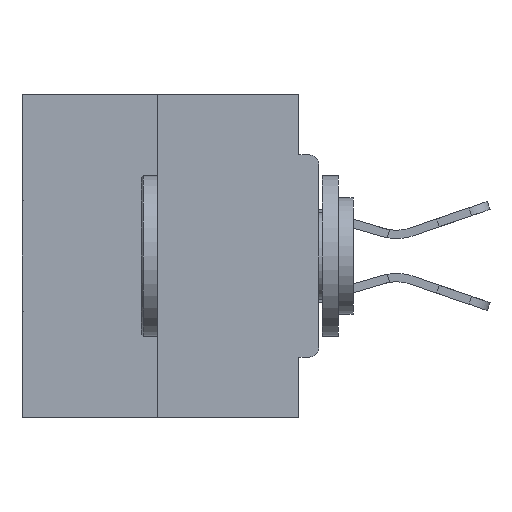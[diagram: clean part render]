
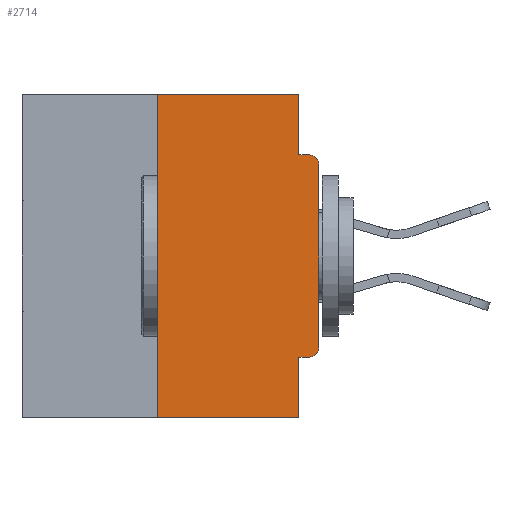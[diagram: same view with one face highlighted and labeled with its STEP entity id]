
A CAD part, left-side view. The second image highlights one B-rep face of the part: STEP entity #2714.
In plain terms, the highlighted planar face has unit normal (-1, 0, 0).
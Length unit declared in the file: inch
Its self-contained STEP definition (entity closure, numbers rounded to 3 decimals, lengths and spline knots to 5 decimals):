
#482 = CARTESIAN_POINT ( 'NONE',  ( 0., 0.25, 0. ) ) ;
#554 = LINE ( 'NONE', #13754, #11994 ) ;
#1395 = CARTESIAN_POINT ( 'NONE',  ( 0., 0.031, -0.4065 ) ) ;
#1674 = EDGE_CURVE ( 'NONE', #18976, #32118, #11681, .T. ) ;
#1680 = AXIS2_PLACEMENT_3D ( 'NONE', #21008, #1879, #27408 ) ;
#1879 = DIRECTION ( 'NONE',  ( -1., 0., 0. ) ) ;
#2221 = VECTOR ( 'NONE', #25900, 39.37008 ) ;
#2714 = ADVANCED_FACE ( 'NONE', ( #7146 ), #31697, .F. ) ;
#2907 = DIRECTION ( 'NONE',  ( 0., -1., 0. ) ) ;
#3108 = DIRECTION ( 'NONE',  ( 1., 0., 0. ) ) ;
#3253 = CARTESIAN_POINT ( 'NONE',  ( 0., 0.46, 0. ) ) ;
#4697 = ORIENTED_EDGE ( 'NONE', *, *, #40764, .F. ) ;
#5365 = DIRECTION ( 'NONE',  ( 0., -1., 0. ) ) ;
#6601 = CARTESIAN_POINT ( 'NONE',  ( 0., 0.015, -0.4065 ) ) ;
#7111 = LINE ( 'NONE', #41302, #9567 ) ;
#7146 = FACE_OUTER_BOUND ( 'NONE', #32315, .T. ) ;
#7966 = ORIENTED_EDGE ( 'NONE', *, *, #26265, .T. ) ;
#8937 = CARTESIAN_POINT ( 'NONE',  ( 0., 0., -0.1085 ) ) ;
#9298 = AXIS2_PLACEMENT_3D ( 'NONE', #3253, #3108, #25711 ) ;
#9567 = VECTOR ( 'NONE', #34832, 39.37008 ) ;
#9929 = VERTEX_POINT ( 'NONE', #32147 ) ;
#10637 = VECTOR ( 'NONE', #37928, 39.37008 ) ;
#10678 = EDGE_CURVE ( 'NONE', #16804, #32118, #7111, .T. ) ;
#10732 = VERTEX_POINT ( 'NONE', #6601 ) ;
#11201 = VECTOR ( 'NONE', #12652, 39.37008 ) ;
#11389 = EDGE_CURVE ( 'NONE', #28008, #25278, #20576, .T. ) ;
#11681 = LINE ( 'NONE', #19490, #2221 ) ;
#11994 = VECTOR ( 'NONE', #16995, 39.37008 ) ;
#12652 = DIRECTION ( 'NONE',  ( 0., 0., 1. ) ) ;
#13375 = ORIENTED_EDGE ( 'NONE', *, *, #17230, .F. ) ;
#13578 = ORIENTED_EDGE ( 'NONE', *, *, #16237, .T. ) ;
#13743 = LINE ( 'NONE', #15184, #34253 ) ;
#13754 = CARTESIAN_POINT ( 'NONE',  ( 0., 0.031, 0. ) ) ;
#15120 = VECTOR ( 'NONE', #5365, 39.37008 ) ;
#15184 = CARTESIAN_POINT ( 'NONE',  ( 0., 0., -0.0935 ) ) ;
#16237 = EDGE_CURVE ( 'NONE', #9929, #28008, #32051, .T. ) ;
#16804 = VERTEX_POINT ( 'NONE', #39982 ) ;
#16995 = DIRECTION ( 'NONE',  ( 0., 0., -1. ) ) ;
#17230 = EDGE_CURVE ( 'NONE', #18029, #40065, #554, .T. ) ;
#18029 = VERTEX_POINT ( 'NONE', #18227 ) ;
#18109 = CIRCLE ( 'NONE', #1680, 0.015 ) ;
#18227 = CARTESIAN_POINT ( 'NONE',  ( 0., 0.031, 0. ) ) ;
#18541 = EDGE_CURVE ( 'NONE', #10732, #18976, #21904, .T. ) ;
#18976 = VERTEX_POINT ( 'NONE', #1395 ) ;
#19490 = CARTESIAN_POINT ( 'NONE',  ( 0., 0.031, -0.5 ) ) ;
#20576 = CIRCLE ( 'NONE', #29931, 0.015 ) ;
#21008 = CARTESIAN_POINT ( 'NONE',  ( 0., 0.015, -0.3915 ) ) ;
#21205 = ORIENTED_EDGE ( 'NONE', *, *, #18541, .F. ) ;
#21664 = ORIENTED_EDGE ( 'NONE', *, *, #11389, .T. ) ;
#21696 = CARTESIAN_POINT ( 'NONE',  ( 0., 0.46, 0. ) ) ;
#21904 = LINE ( 'NONE', #39749, #34835 ) ;
#22258 = CARTESIAN_POINT ( 'NONE',  ( 0., 0.015, -0.0935 ) ) ;
#22420 = ORIENTED_EDGE ( 'NONE', *, *, #30897, .F. ) ;
#23133 = LINE ( 'NONE', #21696, #15120 ) ;
#23676 = EDGE_CURVE ( 'NONE', #16804, #34293, #30185, .T. ) ;
#25278 = VERTEX_POINT ( 'NONE', #22258 ) ;
#25711 = DIRECTION ( 'NONE',  ( 0., 0., -1. ) ) ;
#25900 = DIRECTION ( 'NONE',  ( 0., 0., -1. ) ) ;
#26265 = EDGE_CURVE ( 'NONE', #10732, #9929, #18109, .T. ) ;
#27040 = DIRECTION ( 'NONE',  ( 0., 1., 0. ) ) ;
#27408 = DIRECTION ( 'NONE',  ( 0., 0., -1. ) ) ;
#27870 = ORIENTED_EDGE ( 'NONE', *, *, #23676, .F. ) ;
#28008 = VERTEX_POINT ( 'NONE', #8937 ) ;
#29931 = AXIS2_PLACEMENT_3D ( 'NONE', #40256, #33662, #30861 ) ;
#30185 = LINE ( 'NONE', #37947, #11201 ) ;
#30861 = DIRECTION ( 'NONE',  ( 0., 0., -1. ) ) ;
#30897 = EDGE_CURVE ( 'NONE', #40065, #25278, #13743, .T. ) ;
#31697 = PLANE ( 'NONE',  #9298 ) ;
#32051 = LINE ( 'NONE', #40281, #10637 ) ;
#32118 = VERTEX_POINT ( 'NONE', #36932 ) ;
#32147 = CARTESIAN_POINT ( 'NONE',  ( 0., 0., -0.3915 ) ) ;
#32315 = EDGE_LOOP ( 'NONE', ( #4697, #27870, #37665, #36845, #21205, #7966, #13578, #21664, #22420, #13375 ) ) ;
#33662 = DIRECTION ( 'NONE',  ( -1., 0., 0. ) ) ;
#34253 = VECTOR ( 'NONE', #2907, 39.37008 ) ;
#34293 = VERTEX_POINT ( 'NONE', #482 ) ;
#34832 = DIRECTION ( 'NONE',  ( 0., -1., 0. ) ) ;
#34835 = VECTOR ( 'NONE', #27040, 39.37008 ) ;
#36845 = ORIENTED_EDGE ( 'NONE', *, *, #1674, .F. ) ;
#36932 = CARTESIAN_POINT ( 'NONE',  ( 0., 0.031, -0.5 ) ) ;
#37665 = ORIENTED_EDGE ( 'NONE', *, *, #10678, .T. ) ;
#37928 = DIRECTION ( 'NONE',  ( 0., 0., 1. ) ) ;
#37947 = CARTESIAN_POINT ( 'NONE',  ( 0., 0.25, 0. ) ) ;
#39749 = CARTESIAN_POINT ( 'NONE',  ( 0., 0., -0.4065 ) ) ;
#39982 = CARTESIAN_POINT ( 'NONE',  ( 0., 0.25, -0.5 ) ) ;
#40065 = VERTEX_POINT ( 'NONE', #40743 ) ;
#40256 = CARTESIAN_POINT ( 'NONE',  ( 0., 0.015, -0.1085 ) ) ;
#40281 = CARTESIAN_POINT ( 'NONE',  ( 0., 0., 0. ) ) ;
#40743 = CARTESIAN_POINT ( 'NONE',  ( 0., 0.031, -0.0935 ) ) ;
#40764 = EDGE_CURVE ( 'NONE', #34293, #18029, #23133, .T. ) ;
#41302 = CARTESIAN_POINT ( 'NONE',  ( 0., 0.46, -0.5 ) ) ;
